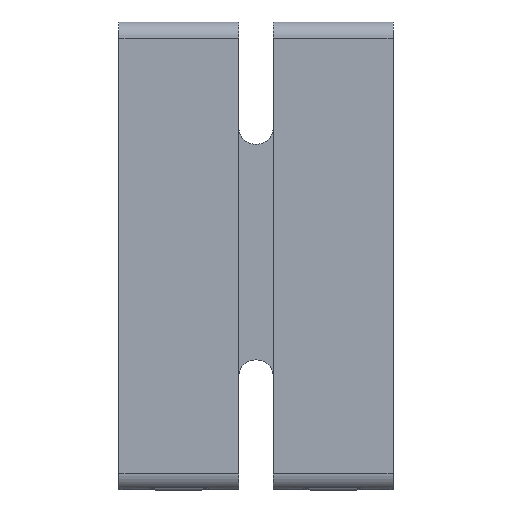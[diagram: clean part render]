
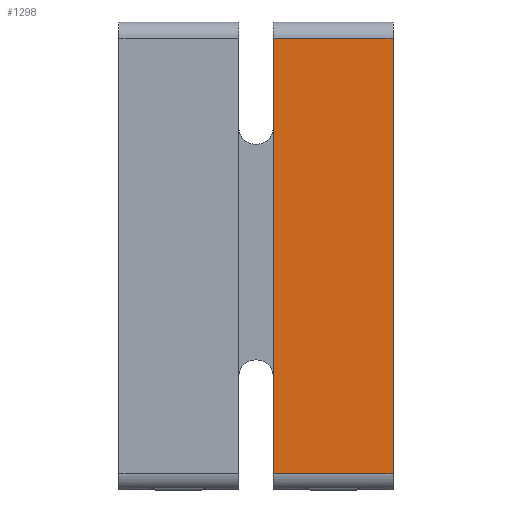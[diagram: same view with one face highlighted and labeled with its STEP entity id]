
A CAD part, front view. The second image highlights one B-rep face of the part: STEP entity #1298.
In plain terms, the highlighted planar face has unit normal (0, -1, 0).
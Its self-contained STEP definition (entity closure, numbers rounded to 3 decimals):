
#160 = VERTEX_POINT ( 'NONE', #1964 ) ;
#192 = CARTESIAN_POINT ( 'NONE',  ( 52.6, -8., 39.64 ) ) ;
#338 = VERTEX_POINT ( 'NONE', #3701 ) ;
#461 = VECTOR ( 'NONE', #3020, 1000. ) ;
#529 = ORIENTED_EDGE ( 'NONE', *, *, #3449, .T. ) ;
#584 = CARTESIAN_POINT ( 'NONE',  ( 3.175, -8., 38.1 ) ) ;
#659 = ORIENTED_EDGE ( 'NONE', *, *, #1170, .T. ) ;
#842 = FACE_OUTER_BOUND ( 'NONE', #2580, .T. ) ;
#1063 = VECTOR ( 'NONE', #2595, 1000. ) ;
#1162 = VERTEX_POINT ( 'NONE', #5136 ) ;
#1170 = EDGE_CURVE ( 'NONE', #5203, #160, #2433, .T. ) ;
#1298 = ADVANCED_FACE ( 'NONE', ( #842 ), #2031, .T. ) ;
#1350 = VECTOR ( 'NONE', #3128, 1000. ) ;
#1377 = CARTESIAN_POINT ( 'NONE',  ( 25.4, -8., -38.1 ) ) ;
#1526 = EDGE_CURVE ( 'NONE', #1162, #338, #2497, .T. ) ;
#1817 = DIRECTION ( 'NONE',  ( 0., 0., -1. ) ) ;
#1964 = CARTESIAN_POINT ( 'NONE',  ( 25.4, -8., -41.1 ) ) ;
#2031 = PLANE ( 'NONE',  #4797 ) ;
#2195 = ORIENTED_EDGE ( 'NONE', *, *, #2464, .T. ) ;
#2424 = CARTESIAN_POINT ( 'NONE',  ( 3.175, -8., -41.1 ) ) ;
#2433 = LINE ( 'NONE', #2713, #1350 ) ;
#2442 = DIRECTION ( 'NONE',  ( 0., 0., -1. ) ) ;
#2464 = EDGE_CURVE ( 'NONE', #338, #5203, #4806, .T. ) ;
#2497 = LINE ( 'NONE', #192, #461 ) ;
#2580 = EDGE_LOOP ( 'NONE', ( #529, #4729, #2195, #659 ) ) ;
#2595 = DIRECTION ( 'NONE',  ( 0., 0., 1. ) ) ;
#2713 = CARTESIAN_POINT ( 'NONE',  ( 0., -8., -41.1 ) ) ;
#3020 = DIRECTION ( 'NONE',  ( -1., 0., 0. ) ) ;
#3128 = DIRECTION ( 'NONE',  ( 1., 0., 0. ) ) ;
#3449 = EDGE_CURVE ( 'NONE', #160, #1162, #4283, .T. ) ;
#3701 = CARTESIAN_POINT ( 'NONE',  ( 3.175, -8., 39.64 ) ) ;
#3737 = VECTOR ( 'NONE', #1817, 1000. ) ;
#4040 = CARTESIAN_POINT ( 'NONE',  ( 0., -8., 0. ) ) ;
#4283 = LINE ( 'NONE', #1377, #1063 ) ;
#4729 = ORIENTED_EDGE ( 'NONE', *, *, #1526, .T. ) ;
#4797 = AXIS2_PLACEMENT_3D ( 'NONE', #4040, #4848, #2442 ) ;
#4806 = LINE ( 'NONE', #584, #3737 ) ;
#4848 = DIRECTION ( 'NONE',  ( 0., -1., 0. ) ) ;
#5136 = CARTESIAN_POINT ( 'NONE',  ( 25.4, -8., 39.64 ) ) ;
#5203 = VERTEX_POINT ( 'NONE', #2424 ) ;
